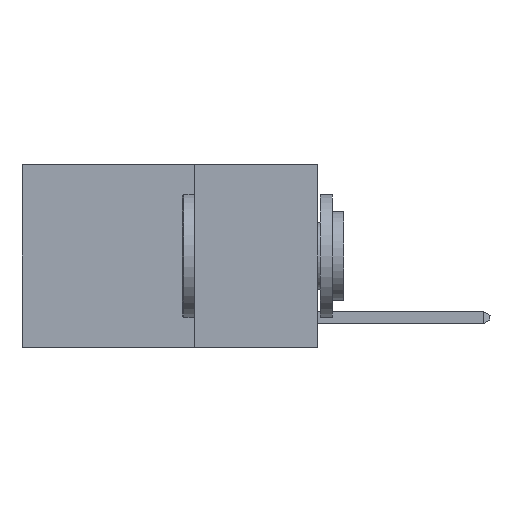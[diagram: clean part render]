
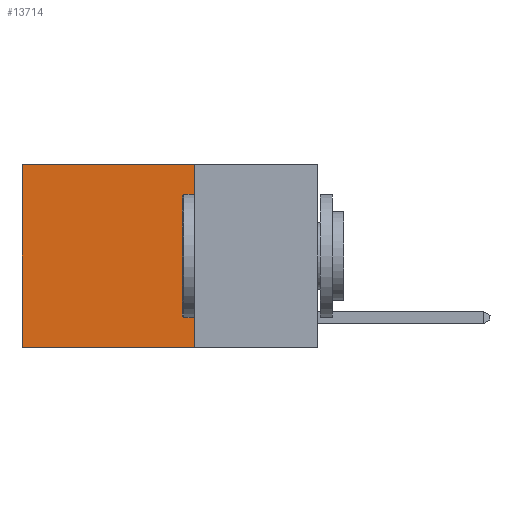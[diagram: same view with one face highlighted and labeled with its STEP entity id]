
A CAD part, left-side view. The second image highlights one B-rep face of the part: STEP entity #13714.
In plain terms, the highlighted planar face has unit normal (-1, 0, 0).
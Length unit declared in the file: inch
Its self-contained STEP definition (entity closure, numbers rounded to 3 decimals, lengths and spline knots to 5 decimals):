
#372 = VERTEX_POINT ( 'NONE', #13120 ) ;
#587 = CARTESIAN_POINT ( 'NONE',  ( 0.2625, 0.25, 0. ) ) ;
#2003 = DIRECTION ( 'NONE',  ( 0., 1., 0. ) ) ;
#2608 = LINE ( 'NONE', #12022, #8902 ) ;
#3326 = ORIENTED_EDGE ( 'NONE', *, *, #14052, .F. ) ;
#3339 = CARTESIAN_POINT ( 'NONE',  ( 0.2625, 0.6, 0. ) ) ;
#3429 = LINE ( 'NONE', #587, #15627 ) ;
#4012 = ORIENTED_EDGE ( 'NONE', *, *, #11259, .T. ) ;
#4084 = VERTEX_POINT ( 'NONE', #15885 ) ;
#4341 = ORIENTED_EDGE ( 'NONE', *, *, #7965, .F. ) ;
#5502 = VECTOR ( 'NONE', #15829, 39.37008 ) ;
#5770 = PLANE ( 'NONE',  #9803 ) ;
#6067 = FACE_OUTER_BOUND ( 'NONE', #10647, .T. ) ;
#7007 = DIRECTION ( 'NONE',  ( 0., 0., -1. ) ) ;
#7545 = VERTEX_POINT ( 'NONE', #14983 ) ;
#7965 = EDGE_CURVE ( 'NONE', #372, #4084, #12139, .T. ) ;
#8338 = DIRECTION ( 'NONE',  ( 0., 0., -1. ) ) ;
#8341 = VERTEX_POINT ( 'NONE', #11099 ) ;
#8483 = ORIENTED_EDGE ( 'NONE', *, *, #8674, .T. ) ;
#8674 = EDGE_CURVE ( 'NONE', #8341, #4084, #9647, .T. ) ;
#8902 = VECTOR ( 'NONE', #8338, 39.37008 ) ;
#9454 = DIRECTION ( 'NONE',  ( 1., 0., 0. ) ) ;
#9647 = LINE ( 'NONE', #3339, #13530 ) ;
#9803 = AXIS2_PLACEMENT_3D ( 'NONE', #15703, #9454, #10779 ) ;
#10647 = EDGE_LOOP ( 'NONE', ( #8483, #4341, #3326, #4012 ) ) ;
#10779 = DIRECTION ( 'NONE',  ( 0., 0., -1. ) ) ;
#11099 = CARTESIAN_POINT ( 'NONE',  ( 0.2625, 0.6, 0. ) ) ;
#11259 = EDGE_CURVE ( 'NONE', #7545, #8341, #3429, .T. ) ;
#12022 = CARTESIAN_POINT ( 'NONE',  ( 0.2625, 0.25, 0. ) ) ;
#12139 = LINE ( 'NONE', #14560, #5502 ) ;
#13120 = CARTESIAN_POINT ( 'NONE',  ( 0.2625, 0.25, -0.37 ) ) ;
#13530 = VECTOR ( 'NONE', #7007, 39.37008 ) ;
#13714 = ADVANCED_FACE ( 'NONE', ( #6067 ), #5770, .F. ) ;
#14052 = EDGE_CURVE ( 'NONE', #7545, #372, #2608, .T. ) ;
#14560 = CARTESIAN_POINT ( 'NONE',  ( 0.2625, 0.25, -0.37 ) ) ;
#14983 = CARTESIAN_POINT ( 'NONE',  ( 0.2625, 0.25, 0. ) ) ;
#15627 = VECTOR ( 'NONE', #2003, 39.37008 ) ;
#15703 = CARTESIAN_POINT ( 'NONE',  ( 0.2625, 0.25, 0. ) ) ;
#15829 = DIRECTION ( 'NONE',  ( 0., 1., 0. ) ) ;
#15885 = CARTESIAN_POINT ( 'NONE',  ( 0.2625, 0.6, -0.37 ) ) ;
